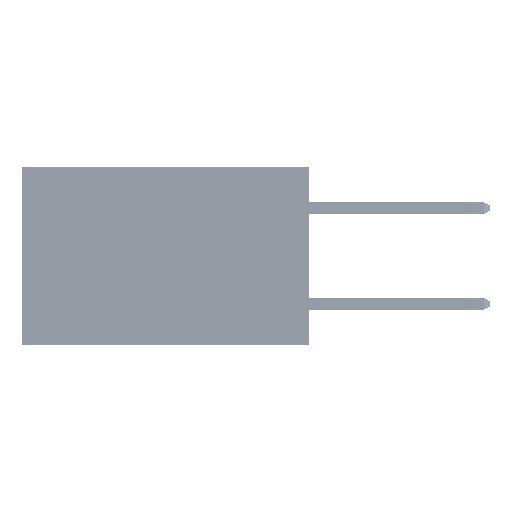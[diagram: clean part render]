
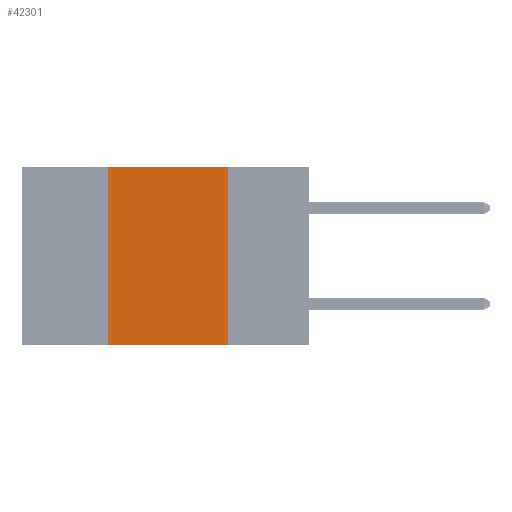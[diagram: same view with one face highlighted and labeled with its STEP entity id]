
A CAD part, left-side view. The second image highlights one B-rep face of the part: STEP entity #42301.
In plain terms, the highlighted planar face has unit normal (-1, 0, 0).
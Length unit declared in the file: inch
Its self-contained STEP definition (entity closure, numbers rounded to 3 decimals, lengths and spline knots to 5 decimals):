
#485 = EDGE_CURVE ( 'NONE', #2994, #36318, #33066, .T. ) ;
#1267 = ORIENTED_EDGE ( 'NONE', *, *, #44915, .F. ) ;
#2994 = VERTEX_POINT ( 'NONE', #20704 ) ;
#5482 = CARTESIAN_POINT ( 'NONE',  ( 0., 0.17, 0. ) ) ;
#6000 = CARTESIAN_POINT ( 'NONE',  ( 0., 0.6, -0.37 ) ) ;
#6065 = ORIENTED_EDGE ( 'NONE', *, *, #31592, .F. ) ;
#6492 = VERTEX_POINT ( 'NONE', #32078 ) ;
#7303 = PLANE ( 'NONE',  #48425 ) ;
#9993 = LINE ( 'NONE', #6000, #49622 ) ;
#12413 = DIRECTION ( 'NONE',  ( 0., 0., 1. ) ) ;
#12734 = EDGE_LOOP ( 'NONE', ( #6065, #31758, #1267, #44755 ) ) ;
#14278 = CARTESIAN_POINT ( 'NONE',  ( 0., 0.17, 0. ) ) ;
#16230 = CARTESIAN_POINT ( 'NONE',  ( 0., 0.6, 0. ) ) ;
#18044 = DIRECTION ( 'NONE',  ( 0., -1., 0. ) ) ;
#19782 = VECTOR ( 'NONE', #12413, 39.37008 ) ;
#20704 = CARTESIAN_POINT ( 'NONE',  ( 0., 0.42, 0. ) ) ;
#22585 = VECTOR ( 'NONE', #24621, 39.37008 ) ;
#24621 = DIRECTION ( 'NONE',  ( 0., -1., 0. ) ) ;
#29238 = LINE ( 'NONE', #5482, #47362 ) ;
#31592 = EDGE_CURVE ( 'NONE', #36318, #36418, #29238, .T. ) ;
#31758 = ORIENTED_EDGE ( 'NONE', *, *, #485, .F. ) ;
#32078 = CARTESIAN_POINT ( 'NONE',  ( 0., 0.42, -0.37 ) ) ;
#33066 = LINE ( 'NONE', #33098, #22585 ) ;
#33098 = CARTESIAN_POINT ( 'NONE',  ( 0., 0.6, 0. ) ) ;
#35053 = EDGE_CURVE ( 'NONE', #6492, #36418, #9993, .T. ) ;
#36318 = VERTEX_POINT ( 'NONE', #14278 ) ;
#36418 = VERTEX_POINT ( 'NONE', #44023 ) ;
#41863 = LINE ( 'NONE', #49604, #19782 ) ;
#42301 = ADVANCED_FACE ( 'NONE', ( #47965 ), #7303, .F. ) ;
#42919 = DIRECTION ( 'NONE',  ( 0., 0., -1. ) ) ;
#44023 = CARTESIAN_POINT ( 'NONE',  ( 0., 0.17, -0.37 ) ) ;
#44755 = ORIENTED_EDGE ( 'NONE', *, *, #35053, .T. ) ;
#44896 = DIRECTION ( 'NONE',  ( 1., 0., 0. ) ) ;
#44915 = EDGE_CURVE ( 'NONE', #6492, #2994, #41863, .T. ) ;
#47362 = VECTOR ( 'NONE', #42919, 39.37008 ) ;
#47965 = FACE_OUTER_BOUND ( 'NONE', #12734, .T. ) ;
#48425 = AXIS2_PLACEMENT_3D ( 'NONE', #16230, #44896, #49593 ) ;
#49593 = DIRECTION ( 'NONE',  ( 0., 0., -1. ) ) ;
#49604 = CARTESIAN_POINT ( 'NONE',  ( 0., 0.42, 0. ) ) ;
#49622 = VECTOR ( 'NONE', #18044, 39.37008 ) ;
